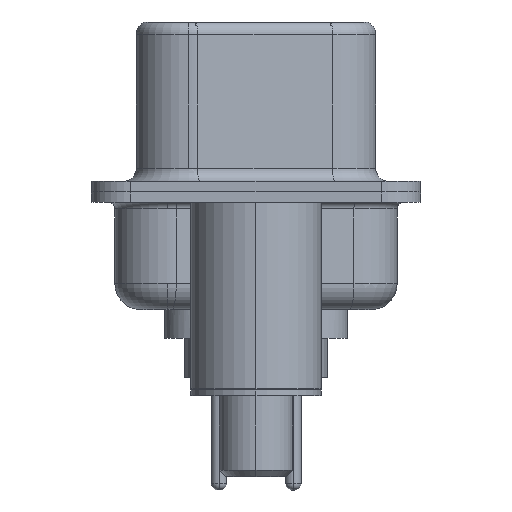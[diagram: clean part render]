
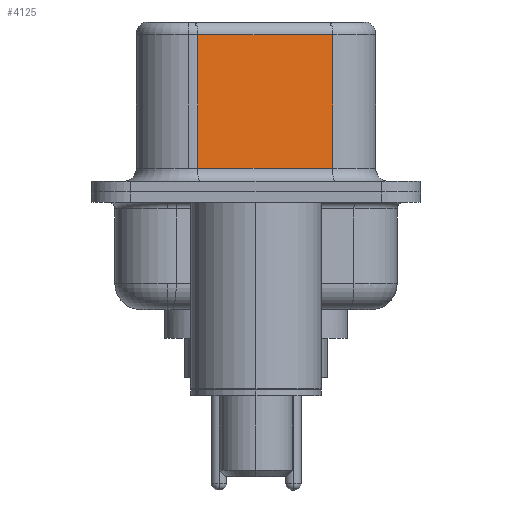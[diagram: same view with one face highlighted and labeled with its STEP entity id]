
A CAD part, left-side view. The second image highlights one B-rep face of the part: STEP entity #4125.
In plain terms, the highlighted planar face has unit normal (-0.985, -0.174, 0).
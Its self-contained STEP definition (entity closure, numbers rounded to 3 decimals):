
#686 = CARTESIAN_POINT ( 'NONE',  ( 4.58, -2.927, 0.9 ) ) ;
#1257 = EDGE_CURVE ( 'NONE', #1621, #20807, #8064, .T. ) ;
#1621 = VERTEX_POINT ( 'NONE', #4069 ) ;
#1794 = EDGE_LOOP ( 'NONE', ( #11023, #8484, #16002, #11041 ) ) ;
#3192 = FACE_OUTER_BOUND ( 'NONE', #1794, .T. ) ;
#3448 = VECTOR ( 'NONE', #21251, 1000. ) ;
#3619 = VECTOR ( 'NONE', #14976, 1000. ) ;
#3641 = CARTESIAN_POINT ( 'NONE',  ( 4.58, -2.927, 6.52 ) ) ;
#4069 = CARTESIAN_POINT ( 'NONE',  ( 4.58, -2.927, 6.02 ) ) ;
#4070 = VERTEX_POINT ( 'NONE', #13495 ) ;
#4125 = ADVANCED_FACE ( 'NONE', ( #3192 ), #11408, .F. ) ;
#4523 = DIRECTION ( 'NONE',  ( 0., 0., -1. ) ) ;
#4662 = CARTESIAN_POINT ( 'NONE',  ( 4.58, -2.927, 6.52 ) ) ;
#5017 = LINE ( 'NONE', #4662, #9621 ) ;
#5541 = EDGE_CURVE ( 'NONE', #1621, #12617, #5017, .T. ) ;
#5917 = EDGE_CURVE ( 'NONE', #20807, #4070, #21711, .T. ) ;
#8064 = LINE ( 'NONE', #12944, #3448 ) ;
#8161 = EDGE_CURVE ( 'NONE', #4070, #12617, #10658, .T. ) ;
#8484 = ORIENTED_EDGE ( 'NONE', *, *, #1257, .T. ) ;
#9621 = VECTOR ( 'NONE', #4523, 1000. ) ;
#10059 = CARTESIAN_POINT ( 'NONE',  ( 4.58, -2.927, 0.9 ) ) ;
#10247 = DIRECTION ( 'NONE',  ( 0.174, -0.985, 0. ) ) ;
#10658 = LINE ( 'NONE', #10059, #19087 ) ;
#10664 = DIRECTION ( 'NONE',  ( 0.985, 0.174, 0. ) ) ;
#10861 = DIRECTION ( 'NONE',  ( -0.174, 0.985, 0. ) ) ;
#11023 = ORIENTED_EDGE ( 'NONE', *, *, #5541, .F. ) ;
#11041 = ORIENTED_EDGE ( 'NONE', *, *, #8161, .T. ) ;
#11408 = PLANE ( 'NONE',  #21494 ) ;
#12617 = VERTEX_POINT ( 'NONE', #686 ) ;
#12944 = CARTESIAN_POINT ( 'NONE',  ( 4.58, -2.927, 6.02 ) ) ;
#13101 = CARTESIAN_POINT ( 'NONE',  ( 3.67, 2.233, 6.02 ) ) ;
#13495 = CARTESIAN_POINT ( 'NONE',  ( 3.67, 2.233, 0.9 ) ) ;
#14976 = DIRECTION ( 'NONE',  ( 0., 0., -1. ) ) ;
#16002 = ORIENTED_EDGE ( 'NONE', *, *, #5917, .T. ) ;
#16201 = CARTESIAN_POINT ( 'NONE',  ( 3.67, 2.233, 6.52 ) ) ;
#19087 = VECTOR ( 'NONE', #10247, 1000. ) ;
#20807 = VERTEX_POINT ( 'NONE', #13101 ) ;
#21251 = DIRECTION ( 'NONE',  ( -0.174, 0.985, 0. ) ) ;
#21494 = AXIS2_PLACEMENT_3D ( 'NONE', #3641, #10664, #10861 ) ;
#21711 = LINE ( 'NONE', #16201, #3619 ) ;
